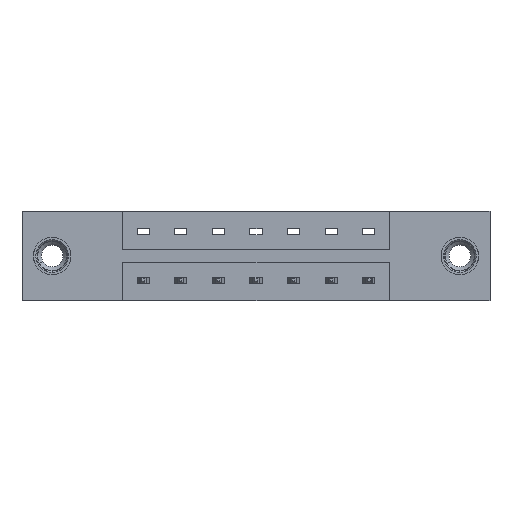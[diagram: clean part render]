
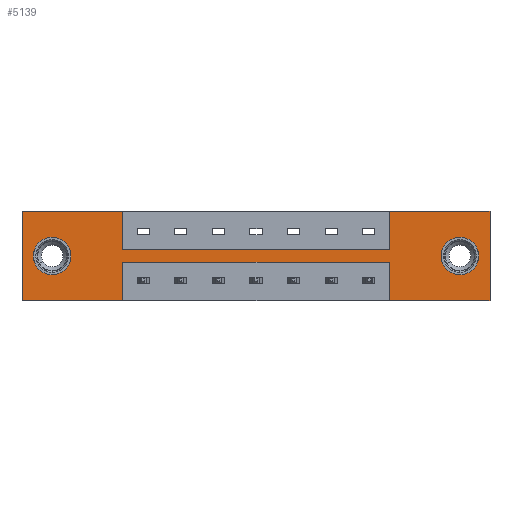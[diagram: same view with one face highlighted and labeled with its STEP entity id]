
A CAD part, front view. The second image highlights one B-rep face of the part: STEP entity #5139.
In plain terms, the highlighted planar face has unit normal (0, -1, 0).
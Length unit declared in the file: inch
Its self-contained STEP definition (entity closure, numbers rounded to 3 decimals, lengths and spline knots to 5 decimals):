
#22 = CARTESIAN_POINT ( 'NONE',  ( 0.125, 0., -0.185 ) ) ;
#34 = ORIENTED_EDGE ( 'NONE', *, *, #5952, .F. ) ;
#71 = ORIENTED_EDGE ( 'NONE', *, *, #5270, .F. ) ;
#98 = VERTEX_POINT ( 'NONE', #7702 ) ;
#175 = CIRCLE ( 'NONE', #7305, 0.078 ) ;
#364 = LINE ( 'NONE', #415, #5929 ) ;
#387 = LINE ( 'NONE', #3477, #3933 ) ;
#415 = CARTESIAN_POINT ( 'NONE',  ( 0.4175, 0., -0.2115 ) ) ;
#474 = CARTESIAN_POINT ( 'NONE',  ( 0.4175, 0., -0.2115 ) ) ;
#572 = CARTESIAN_POINT ( 'NONE',  ( 0., 0., 0. ) ) ;
#802 = CARTESIAN_POINT ( 'NONE',  ( 1.815, 0., -0.107 ) ) ;
#1003 = DIRECTION ( 'NONE',  ( 0., 1., 0. ) ) ;
#1028 = LINE ( 'NONE', #2451, #3586 ) ;
#1075 = DIRECTION ( 'NONE',  ( 0., 1., 0. ) ) ;
#1083 = CARTESIAN_POINT ( 'NONE',  ( 1.5225, 0., 0. ) ) ;
#1089 = VERTEX_POINT ( 'NONE', #4061 ) ;
#1095 = ORIENTED_EDGE ( 'NONE', *, *, #3503, .F. ) ;
#1171 = EDGE_CURVE ( 'NONE', #4260, #2205, #364, .T. ) ;
#1204 = VERTEX_POINT ( 'NONE', #2021 ) ;
#1219 = DIRECTION ( 'NONE',  ( 0., 0., -1. ) ) ;
#1273 = ORIENTED_EDGE ( 'NONE', *, *, #7655, .T. ) ;
#1421 = ORIENTED_EDGE ( 'NONE', *, *, #2825, .T. ) ;
#1499 = VERTEX_POINT ( 'NONE', #9626 ) ;
#1534 = DIRECTION ( 'NONE',  ( 0., 0., -1. ) ) ;
#1632 = PLANE ( 'NONE',  #5461 ) ;
#1683 = FACE_BOUND ( 'NONE', #9281, .T. ) ;
#1720 = LINE ( 'NONE', #7976, #2608 ) ;
#1759 = VECTOR ( 'NONE', #7717, 39.37008 ) ;
#1763 = CARTESIAN_POINT ( 'NONE',  ( 1.815, 0., -0.185 ) ) ;
#1814 = ORIENTED_EDGE ( 'NONE', *, *, #1171, .F. ) ;
#1861 = CARTESIAN_POINT ( 'NONE',  ( 1.815, 0., -0.263 ) ) ;
#1981 = CARTESIAN_POINT ( 'NONE',  ( 1.5225, 0., -0.2115 ) ) ;
#2009 = ORIENTED_EDGE ( 'NONE', *, *, #6772, .F. ) ;
#2015 = DIRECTION ( 'NONE',  ( 0., 0., 1. ) ) ;
#2021 = CARTESIAN_POINT ( 'NONE',  ( 0.4175, 0., 0. ) ) ;
#2113 = VERTEX_POINT ( 'NONE', #6789 ) ;
#2168 = LINE ( 'NONE', #572, #1759 ) ;
#2205 = VERTEX_POINT ( 'NONE', #7449 ) ;
#2393 = CARTESIAN_POINT ( 'NONE',  ( 0., 0., -0.37 ) ) ;
#2450 = FACE_BOUND ( 'NONE', #9993, .T. ) ;
#2451 = CARTESIAN_POINT ( 'NONE',  ( 0.4175, 0., -0.2115 ) ) ;
#2458 = LINE ( 'NONE', #6227, #6193 ) ;
#2496 = DIRECTION ( 'NONE',  ( 0., 0., -1. ) ) ;
#2587 = DIRECTION ( 'NONE',  ( -1., 0., 0. ) ) ;
#2608 = VECTOR ( 'NONE', #2587, 39.37008 ) ;
#2653 = DIRECTION ( 'NONE',  ( -1., 0., 0. ) ) ;
#2798 = ORIENTED_EDGE ( 'NONE', *, *, #7507, .F. ) ;
#2810 = EDGE_CURVE ( 'NONE', #2205, #2113, #1720, .T. ) ;
#2825 = EDGE_CURVE ( 'NONE', #9138, #4729, #5531, .T. ) ;
#2843 = CARTESIAN_POINT ( 'NONE',  ( 1.94, 0., 0. ) ) ;
#3057 = CARTESIAN_POINT ( 'NONE',  ( 0., 0., 0. ) ) ;
#3109 = LINE ( 'NONE', #9360, #9900 ) ;
#3204 = VERTEX_POINT ( 'NONE', #7409 ) ;
#3223 = EDGE_CURVE ( 'NONE', #4786, #4202, #4967, .T. ) ;
#3405 = CIRCLE ( 'NONE', #4542, 0.078 ) ;
#3477 = CARTESIAN_POINT ( 'NONE',  ( 0., 0., 0. ) ) ;
#3503 = EDGE_CURVE ( 'NONE', #1204, #1089, #2458, .T. ) ;
#3586 = VECTOR ( 'NONE', #2653, 39.37008 ) ;
#3800 = ORIENTED_EDGE ( 'NONE', *, *, #6400, .T. ) ;
#3810 = EDGE_CURVE ( 'NONE', #4599, #3204, #5396, .T. ) ;
#3890 = VECTOR ( 'NONE', #4792, 39.37008 ) ;
#3933 = VECTOR ( 'NONE', #4282, 39.37008 ) ;
#4025 = DIRECTION ( 'NONE',  ( 0., 1., 0. ) ) ;
#4061 = CARTESIAN_POINT ( 'NONE',  ( 0.4175, 0., -0.1585 ) ) ;
#4102 = ORIENTED_EDGE ( 'NONE', *, *, #8367, .F. ) ;
#4176 = DIRECTION ( 'NONE',  ( 0., 0., -1. ) ) ;
#4201 = DIRECTION ( 'NONE',  ( 0., 0., 1. ) ) ;
#4202 = VERTEX_POINT ( 'NONE', #1981 ) ;
#4260 = VERTEX_POINT ( 'NONE', #474 ) ;
#4264 = ORIENTED_EDGE ( 'NONE', *, *, #2810, .F. ) ;
#4282 = DIRECTION ( 'NONE',  ( 1., 0., 0. ) ) ;
#4542 = AXIS2_PLACEMENT_3D ( 'NONE', #8716, #1003, #2015 ) ;
#4577 = LINE ( 'NONE', #3057, #9737 ) ;
#4599 = VERTEX_POINT ( 'NONE', #2843 ) ;
#4650 = DIRECTION ( 'NONE',  ( 0., 0., -1. ) ) ;
#4716 = CARTESIAN_POINT ( 'NONE',  ( 1.5225, 0., -0.1585 ) ) ;
#4729 = VERTEX_POINT ( 'NONE', #802 ) ;
#4786 = VERTEX_POINT ( 'NONE', #6245 ) ;
#4792 = DIRECTION ( 'NONE',  ( 0., 0., 1. ) ) ;
#4934 = DIRECTION ( 'NONE',  ( 1., 0., 0. ) ) ;
#4967 = LINE ( 'NONE', #9726, #9602 ) ;
#4984 = CIRCLE ( 'NONE', #8592, 0.078 ) ;
#5139 = ADVANCED_FACE ( 'NONE', ( #2450, #1683, #8541 ), #1632, .T. ) ;
#5225 = EDGE_CURVE ( 'NONE', #98, #8639, #4984, .T. ) ;
#5236 = DIRECTION ( 'NONE',  ( -1., 0., 0. ) ) ;
#5270 = EDGE_CURVE ( 'NONE', #7619, #6753, #5450, .T. ) ;
#5396 = LINE ( 'NONE', #7031, #7180 ) ;
#5450 = LINE ( 'NONE', #7127, #3890 ) ;
#5461 = AXIS2_PLACEMENT_3D ( 'NONE', #2393, #6214, #1534 ) ;
#5531 = CIRCLE ( 'NONE', #9428, 0.078 ) ;
#5722 = DIRECTION ( 'NONE',  ( 0., 0., -1. ) ) ;
#5929 = VECTOR ( 'NONE', #1219, 39.37008 ) ;
#5952 = EDGE_CURVE ( 'NONE', #3204, #4786, #8276, .T. ) ;
#6160 = DIRECTION ( 'NONE',  ( 0., 0., 1. ) ) ;
#6193 = VECTOR ( 'NONE', #4650, 39.37008 ) ;
#6214 = DIRECTION ( 'NONE',  ( 0., -1., 0. ) ) ;
#6227 = CARTESIAN_POINT ( 'NONE',  ( 0.4175, 0., -0.1585 ) ) ;
#6245 = CARTESIAN_POINT ( 'NONE',  ( 1.5225, 0., -0.37 ) ) ;
#6400 = EDGE_CURVE ( 'NONE', #4729, #9138, #175, .T. ) ;
#6437 = ORIENTED_EDGE ( 'NONE', *, *, #3810, .F. ) ;
#6598 = ORIENTED_EDGE ( 'NONE', *, *, #3223, .F. ) ;
#6753 = VERTEX_POINT ( 'NONE', #1083 ) ;
#6772 = EDGE_CURVE ( 'NONE', #4202, #4260, #1028, .T. ) ;
#6789 = CARTESIAN_POINT ( 'NONE',  ( 0., 0., -0.37 ) ) ;
#7031 = CARTESIAN_POINT ( 'NONE',  ( 1.94, 0., 0. ) ) ;
#7127 = CARTESIAN_POINT ( 'NONE',  ( 1.5225, 0., -0.1585 ) ) ;
#7180 = VECTOR ( 'NONE', #2496, 39.37008 ) ;
#7243 = CARTESIAN_POINT ( 'NONE',  ( 1.815, 0., -0.185 ) ) ;
#7305 = AXIS2_PLACEMENT_3D ( 'NONE', #7243, #8053, #5722 ) ;
#7409 = CARTESIAN_POINT ( 'NONE',  ( 1.94, 0., -0.37 ) ) ;
#7449 = CARTESIAN_POINT ( 'NONE',  ( 0.4175, 0., -0.37 ) ) ;
#7507 = EDGE_CURVE ( 'NONE', #2113, #1499, #2168, .T. ) ;
#7619 = VERTEX_POINT ( 'NONE', #4716 ) ;
#7655 = EDGE_CURVE ( 'NONE', #8639, #98, #3405, .T. ) ;
#7702 = CARTESIAN_POINT ( 'NONE',  ( 0.125, 0., -0.263 ) ) ;
#7717 = DIRECTION ( 'NONE',  ( 0., 0., 1. ) ) ;
#7871 = EDGE_LOOP ( 'NONE', ( #6598, #34, #6437, #9488, #71, #4102, #1095, #8808, #2798, #4264, #1814, #2009 ) ) ;
#7976 = CARTESIAN_POINT ( 'NONE',  ( 0., 0., -0.37 ) ) ;
#8053 = DIRECTION ( 'NONE',  ( 0., 1., 0. ) ) ;
#8276 = LINE ( 'NONE', #9039, #8749 ) ;
#8367 = EDGE_CURVE ( 'NONE', #1089, #7619, #3109, .T. ) ;
#8427 = EDGE_CURVE ( 'NONE', #1499, #1204, #4577, .T. ) ;
#8541 = FACE_OUTER_BOUND ( 'NONE', #7871, .T. ) ;
#8578 = DIRECTION ( 'NONE',  ( 1., 0., 0. ) ) ;
#8592 = AXIS2_PLACEMENT_3D ( 'NONE', #22, #4025, #6160 ) ;
#8639 = VERTEX_POINT ( 'NONE', #8887 ) ;
#8716 = CARTESIAN_POINT ( 'NONE',  ( 0.125, 0., -0.185 ) ) ;
#8749 = VECTOR ( 'NONE', #5236, 39.37008 ) ;
#8808 = ORIENTED_EDGE ( 'NONE', *, *, #8427, .F. ) ;
#8831 = ORIENTED_EDGE ( 'NONE', *, *, #5225, .T. ) ;
#8887 = CARTESIAN_POINT ( 'NONE',  ( 0.125, 0., -0.107 ) ) ;
#9039 = CARTESIAN_POINT ( 'NONE',  ( 0., 0., -0.37 ) ) ;
#9138 = VERTEX_POINT ( 'NONE', #1861 ) ;
#9281 = EDGE_LOOP ( 'NONE', ( #1273, #8831 ) ) ;
#9360 = CARTESIAN_POINT ( 'NONE',  ( 0.4175, 0., -0.1585 ) ) ;
#9428 = AXIS2_PLACEMENT_3D ( 'NONE', #1763, #1075, #4176 ) ;
#9488 = ORIENTED_EDGE ( 'NONE', *, *, #9877, .F. ) ;
#9602 = VECTOR ( 'NONE', #4201, 39.37008 ) ;
#9626 = CARTESIAN_POINT ( 'NONE',  ( 0., 0., 0. ) ) ;
#9726 = CARTESIAN_POINT ( 'NONE',  ( 1.5225, 0., -0.2115 ) ) ;
#9737 = VECTOR ( 'NONE', #4934, 39.37008 ) ;
#9877 = EDGE_CURVE ( 'NONE', #6753, #4599, #387, .T. ) ;
#9900 = VECTOR ( 'NONE', #8578, 39.37008 ) ;
#9993 = EDGE_LOOP ( 'NONE', ( #3800, #1421 ) ) ;
